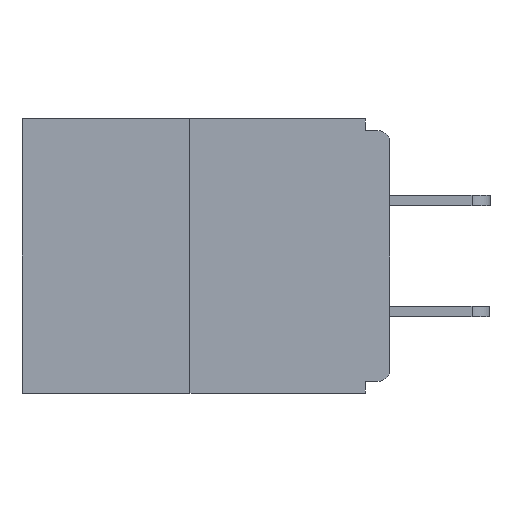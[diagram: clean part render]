
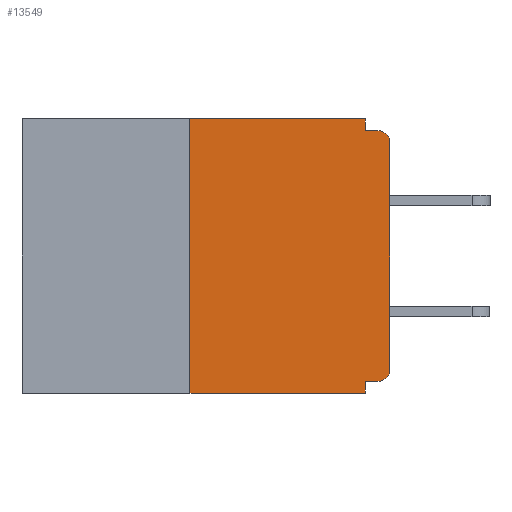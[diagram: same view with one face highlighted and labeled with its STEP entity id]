
A CAD part, left-side view. The second image highlights one B-rep face of the part: STEP entity #13549.
In plain terms, the highlighted planar face has unit normal (-1, 0, 0).
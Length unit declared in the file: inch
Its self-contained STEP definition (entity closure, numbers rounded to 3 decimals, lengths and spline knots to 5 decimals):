
#108 = DIRECTION ( 'NONE',  ( 0., 0., 1. ) ) ;
#319 = CARTESIAN_POINT ( 'NONE',  ( 0., 0., -0.313 ) ) ;
#403 = ORIENTED_EDGE ( 'NONE', *, *, #3472, .F. ) ;
#446 = VECTOR ( 'NONE', #17239, 39.37008 ) ;
#584 = VECTOR ( 'NONE', #108, 39.37008 ) ;
#686 = VERTEX_POINT ( 'NONE', #15505 ) ;
#1082 = VERTEX_POINT ( 'NONE', #9927 ) ;
#1738 = EDGE_LOOP ( 'NONE', ( #12804, #9256, #6143, #2548, #403, #6848, #12684, #2930, #1936, #2344 ) ) ;
#1936 = ORIENTED_EDGE ( 'NONE', *, *, #6105, .F. ) ;
#1964 = CARTESIAN_POINT ( 'NONE',  ( 0., 0.015, -0.313 ) ) ;
#1989 = LINE ( 'NONE', #15213, #8932 ) ;
#2069 = CARTESIAN_POINT ( 'NONE',  ( 0., 0.031, -0.343 ) ) ;
#2192 = DIRECTION ( 'NONE',  ( -1., 0., 0. ) ) ;
#2344 = ORIENTED_EDGE ( 'NONE', *, *, #7022, .F. ) ;
#2548 = ORIENTED_EDGE ( 'NONE', *, *, #9232, .F. ) ;
#2930 = ORIENTED_EDGE ( 'NONE', *, *, #11412, .T. ) ;
#2989 = CARTESIAN_POINT ( 'NONE',  ( 0., 0., 0. ) ) ;
#3250 = LINE ( 'NONE', #2069, #11909 ) ;
#3472 = EDGE_CURVE ( 'NONE', #8005, #15768, #1989, .T. ) ;
#3568 = DIRECTION ( 'NONE',  ( 0., 0., -1. ) ) ;
#3571 = LINE ( 'NONE', #6534, #446 ) ;
#4234 = DIRECTION ( 'NONE',  ( 0., 0., -1. ) ) ;
#4340 = EDGE_CURVE ( 'NONE', #8005, #6005, #12285, .T. ) ;
#4428 = CARTESIAN_POINT ( 'NONE',  ( 0., 0.031, -0.015 ) ) ;
#4601 = CARTESIAN_POINT ( 'NONE',  ( 0., 0.25, 0. ) ) ;
#4842 = CIRCLE ( 'NONE', #17503, 0.015 ) ;
#4847 = CARTESIAN_POINT ( 'NONE',  ( 0., 0.031, -0.328 ) ) ;
#5213 = LINE ( 'NONE', #14284, #7747 ) ;
#5853 = VECTOR ( 'NONE', #8564, 39.37008 ) ;
#6000 = CARTESIAN_POINT ( 'NONE',  ( 0., 0.015, -0.328 ) ) ;
#6005 = VERTEX_POINT ( 'NONE', #319 ) ;
#6105 = EDGE_CURVE ( 'NONE', #17401, #1082, #10966, .T. ) ;
#6143 = ORIENTED_EDGE ( 'NONE', *, *, #11532, .T. ) ;
#6534 = CARTESIAN_POINT ( 'NONE',  ( 0., 0.46, -0.343 ) ) ;
#6652 = EDGE_CURVE ( 'NONE', #9058, #17445, #15806, .T. ) ;
#6848 = ORIENTED_EDGE ( 'NONE', *, *, #4340, .T. ) ;
#7022 = EDGE_CURVE ( 'NONE', #686, #17401, #7117, .T. ) ;
#7117 = LINE ( 'NONE', #11161, #11738 ) ;
#7207 = CARTESIAN_POINT ( 'NONE',  ( 0., 0.25, 0. ) ) ;
#7471 = AXIS2_PLACEMENT_3D ( 'NONE', #1964, #2192, #10100 ) ;
#7747 = VECTOR ( 'NONE', #12974, 39.37008 ) ;
#7790 = EDGE_CURVE ( 'NONE', #6005, #12872, #13854, .T. ) ;
#8005 = VERTEX_POINT ( 'NONE', #6000 ) ;
#8088 = PLANE ( 'NONE',  #8712 ) ;
#8248 = CARTESIAN_POINT ( 'NONE',  ( 0., 0.015, -0.03 ) ) ;
#8465 = DIRECTION ( 'NONE',  ( 0., 1., 0. ) ) ;
#8490 = DIRECTION ( 'NONE',  ( 0., 0., -1. ) ) ;
#8564 = DIRECTION ( 'NONE',  ( 0., 0., 1. ) ) ;
#8712 = AXIS2_PLACEMENT_3D ( 'NONE', #9375, #10562, #11941 ) ;
#8932 = VECTOR ( 'NONE', #8465, 39.37008 ) ;
#9058 = VERTEX_POINT ( 'NONE', #10614 ) ;
#9232 = EDGE_CURVE ( 'NONE', #15768, #12130, #3250, .T. ) ;
#9256 = ORIENTED_EDGE ( 'NONE', *, *, #6652, .F. ) ;
#9375 = CARTESIAN_POINT ( 'NONE',  ( 0., 0.46, 0. ) ) ;
#9927 = CARTESIAN_POINT ( 'NONE',  ( 0., 0.015, -0.015 ) ) ;
#10100 = DIRECTION ( 'NONE',  ( 0., 0., -1. ) ) ;
#10172 = CARTESIAN_POINT ( 'NONE',  ( 0., 0.031, -0.343 ) ) ;
#10562 = DIRECTION ( 'NONE',  ( 1., 0., 0. ) ) ;
#10614 = CARTESIAN_POINT ( 'NONE',  ( 0., 0.25, -0.343 ) ) ;
#10966 = LINE ( 'NONE', #13809, #15613 ) ;
#11161 = CARTESIAN_POINT ( 'NONE',  ( 0., 0.031, 0. ) ) ;
#11353 = FACE_OUTER_BOUND ( 'NONE', #1738, .T. ) ;
#11412 = EDGE_CURVE ( 'NONE', #12872, #1082, #4842, .T. ) ;
#11532 = EDGE_CURVE ( 'NONE', #9058, #12130, #3571, .T. ) ;
#11738 = VECTOR ( 'NONE', #8490, 39.37008 ) ;
#11909 = VECTOR ( 'NONE', #3568, 39.37008 ) ;
#11941 = DIRECTION ( 'NONE',  ( 0., 0., -1. ) ) ;
#12130 = VERTEX_POINT ( 'NONE', #10172 ) ;
#12285 = CIRCLE ( 'NONE', #7471, 0.015 ) ;
#12331 = DIRECTION ( 'NONE',  ( -1., 0., 0. ) ) ;
#12453 = EDGE_CURVE ( 'NONE', #17445, #686, #5213, .T. ) ;
#12684 = ORIENTED_EDGE ( 'NONE', *, *, #7790, .T. ) ;
#12804 = ORIENTED_EDGE ( 'NONE', *, *, #12453, .F. ) ;
#12872 = VERTEX_POINT ( 'NONE', #12958 ) ;
#12958 = CARTESIAN_POINT ( 'NONE',  ( 0., 0., -0.03 ) ) ;
#12974 = DIRECTION ( 'NONE',  ( 0., -1., 0. ) ) ;
#13549 = ADVANCED_FACE ( 'NONE', ( #11353 ), #8088, .F. ) ;
#13809 = CARTESIAN_POINT ( 'NONE',  ( 0., 0., -0.015 ) ) ;
#13854 = LINE ( 'NONE', #2989, #584 ) ;
#14284 = CARTESIAN_POINT ( 'NONE',  ( 0., 0.46, 0. ) ) ;
#15213 = CARTESIAN_POINT ( 'NONE',  ( 0., 0., -0.328 ) ) ;
#15505 = CARTESIAN_POINT ( 'NONE',  ( 0., 0.031, 0. ) ) ;
#15613 = VECTOR ( 'NONE', #16421, 39.37008 ) ;
#15768 = VERTEX_POINT ( 'NONE', #4847 ) ;
#15806 = LINE ( 'NONE', #7207, #5853 ) ;
#16421 = DIRECTION ( 'NONE',  ( 0., -1., 0. ) ) ;
#17239 = DIRECTION ( 'NONE',  ( 0., -1., 0. ) ) ;
#17401 = VERTEX_POINT ( 'NONE', #4428 ) ;
#17445 = VERTEX_POINT ( 'NONE', #4601 ) ;
#17503 = AXIS2_PLACEMENT_3D ( 'NONE', #8248, #12331, #4234 ) ;
